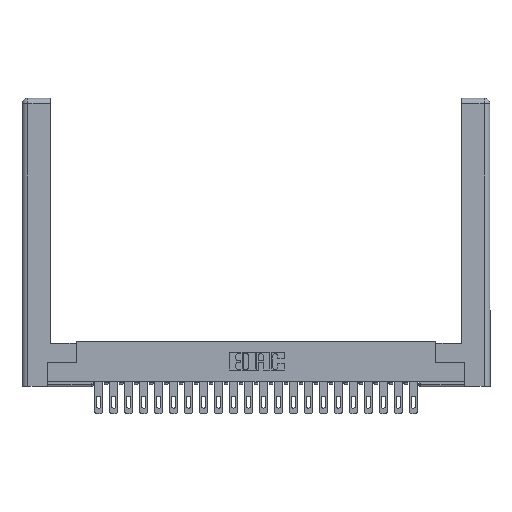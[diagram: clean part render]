
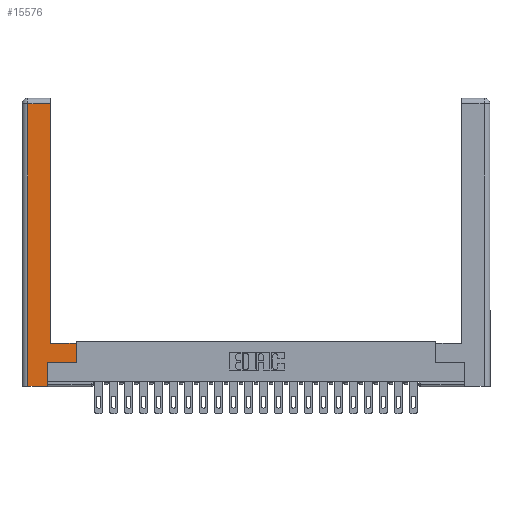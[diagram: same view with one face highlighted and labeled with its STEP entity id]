
A CAD part, top view. The second image highlights one B-rep face of the part: STEP entity #15576.
In plain terms, the highlighted planar face has unit normal (0, 0, 1).
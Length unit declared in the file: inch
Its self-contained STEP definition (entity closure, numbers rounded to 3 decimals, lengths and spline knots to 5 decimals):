
#607 = CARTESIAN_POINT ( 'NONE',  ( 0.565, 0.245, 0. ) ) ;
#985 = DIRECTION ( 'NONE',  ( -1., 0., 0. ) ) ;
#1081 = VERTEX_POINT ( 'NONE', #15176 ) ;
#1765 = CARTESIAN_POINT ( 'NONE',  ( 0.295, 0.45, 0. ) ) ;
#1893 = CARTESIAN_POINT ( 'NONE',  ( 0.565, 0.45, 0. ) ) ;
#1945 = DIRECTION ( 'NONE',  ( 0., 0., -1. ) ) ;
#2283 = AXIS2_PLACEMENT_3D ( 'NONE', #20809, #1945, #14931 ) ;
#2444 = DIRECTION ( 'NONE',  ( 0., 1., 0. ) ) ;
#2654 = CARTESIAN_POINT ( 'NONE',  ( 0.295, 2.94, 0. ) ) ;
#2961 = EDGE_CURVE ( 'NONE', #22816, #14763, #4387, .T. ) ;
#3412 = EDGE_CURVE ( 'NONE', #10032, #5144, #18998, .T. ) ;
#3506 = EDGE_CURVE ( 'NONE', #1081, #22816, #21602, .T. ) ;
#3562 = ORIENTED_EDGE ( 'NONE', *, *, #11510, .T. ) ;
#3576 = PLANE ( 'NONE',  #2283 ) ;
#3982 = CARTESIAN_POINT ( 'NONE',  ( 0.565, 0.45, 0. ) ) ;
#4358 = EDGE_CURVE ( 'NONE', #9518, #24592, #19550, .T. ) ;
#4387 = LINE ( 'NONE', #13900, #24172 ) ;
#4568 = VECTOR ( 'NONE', #985, 39.37008 ) ;
#4962 = ORIENTED_EDGE ( 'NONE', *, *, #6299, .T. ) ;
#5144 = VERTEX_POINT ( 'NONE', #3982 ) ;
#5453 = ORIENTED_EDGE ( 'NONE', *, *, #3506, .T. ) ;
#5841 = ORIENTED_EDGE ( 'NONE', *, *, #17484, .T. ) ;
#6299 = EDGE_CURVE ( 'NONE', #11326, #1081, #8900, .T. ) ;
#6304 = VECTOR ( 'NONE', #9223, 39.37008 ) ;
#6723 = CARTESIAN_POINT ( 'NONE',  ( 0.295, 0.45, 0. ) ) ;
#7857 = ORIENTED_EDGE ( 'NONE', *, *, #2961, .T. ) ;
#8347 = CARTESIAN_POINT ( 'NONE',  ( 0.265, 0., 0. ) ) ;
#8374 = ORIENTED_EDGE ( 'NONE', *, *, #3412, .T. ) ;
#8488 = DIRECTION ( 'NONE',  ( 1., 0., 0. ) ) ;
#8623 = CARTESIAN_POINT ( 'NONE',  ( 0.265, 0., 0. ) ) ;
#8900 = LINE ( 'NONE', #10669, #24091 ) ;
#9223 = DIRECTION ( 'NONE',  ( 1., 0., 0. ) ) ;
#9518 = VERTEX_POINT ( 'NONE', #1765 ) ;
#10032 = VERTEX_POINT ( 'NONE', #607 ) ;
#10669 = CARTESIAN_POINT ( 'NONE',  ( 0.0615, 0., 0. ) ) ;
#10729 = VECTOR ( 'NONE', #21688, 39.37008 ) ;
#11112 = CARTESIAN_POINT ( 'NONE',  ( 0.565, 0.245, 0. ) ) ;
#11273 = CARTESIAN_POINT ( 'NONE',  ( 0.265, 0.245, 0. ) ) ;
#11326 = VERTEX_POINT ( 'NONE', #11384 ) ;
#11384 = CARTESIAN_POINT ( 'NONE',  ( 0.0615, 2.94, 0. ) ) ;
#11474 = VECTOR ( 'NONE', #8488, 39.37008 ) ;
#11510 = EDGE_CURVE ( 'NONE', #5144, #9518, #16453, .T. ) ;
#11737 = CARTESIAN_POINT ( 'NONE',  ( 0.0615, 2.94, 0. ) ) ;
#13900 = CARTESIAN_POINT ( 'NONE',  ( 0.265, 0.245, 0. ) ) ;
#14763 = VERTEX_POINT ( 'NONE', #11273 ) ;
#14931 = DIRECTION ( 'NONE',  ( -1., 0., 0. ) ) ;
#15176 = CARTESIAN_POINT ( 'NONE',  ( 0.0615, 0., 0. ) ) ;
#15247 = DIRECTION ( 'NONE',  ( 0., 1., 0. ) ) ;
#15576 = ADVANCED_FACE ( 'NONE', ( #18802 ), #3576, .F. ) ;
#16010 = ORIENTED_EDGE ( 'NONE', *, *, #4358, .T. ) ;
#16387 = DIRECTION ( 'NONE',  ( 0., -1., 0. ) ) ;
#16453 = LINE ( 'NONE', #6723, #4568 ) ;
#16613 = VECTOR ( 'NONE', #15247, 39.37008 ) ;
#17484 = EDGE_CURVE ( 'NONE', #14763, #10032, #20709, .T. ) ;
#17649 = VECTOR ( 'NONE', #2444, 39.37008 ) ;
#18006 = DIRECTION ( 'NONE',  ( 0., 1., 0. ) ) ;
#18802 = FACE_OUTER_BOUND ( 'NONE', #24120, .T. ) ;
#18933 = ORIENTED_EDGE ( 'NONE', *, *, #22856, .T. ) ;
#18998 = LINE ( 'NONE', #1893, #16613 ) ;
#19550 = LINE ( 'NONE', #19797, #17649 ) ;
#19584 = LINE ( 'NONE', #11737, #10729 ) ;
#19797 = CARTESIAN_POINT ( 'NONE',  ( 0.295, 3., 0. ) ) ;
#20709 = LINE ( 'NONE', #11112, #6304 ) ;
#20809 = CARTESIAN_POINT ( 'NONE',  ( 0., 0., 0. ) ) ;
#21602 = LINE ( 'NONE', #8623, #11474 ) ;
#21688 = DIRECTION ( 'NONE',  ( -1., 0., 0. ) ) ;
#22816 = VERTEX_POINT ( 'NONE', #8347 ) ;
#22856 = EDGE_CURVE ( 'NONE', #24592, #11326, #19584, .T. ) ;
#24091 = VECTOR ( 'NONE', #16387, 39.37008 ) ;
#24120 = EDGE_LOOP ( 'NONE', ( #16010, #18933, #4962, #5453, #7857, #5841, #8374, #3562 ) ) ;
#24172 = VECTOR ( 'NONE', #18006, 39.37008 ) ;
#24592 = VERTEX_POINT ( 'NONE', #2654 ) ;
